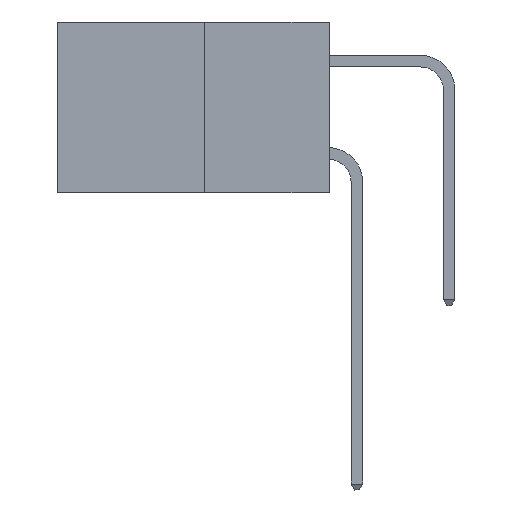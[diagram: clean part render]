
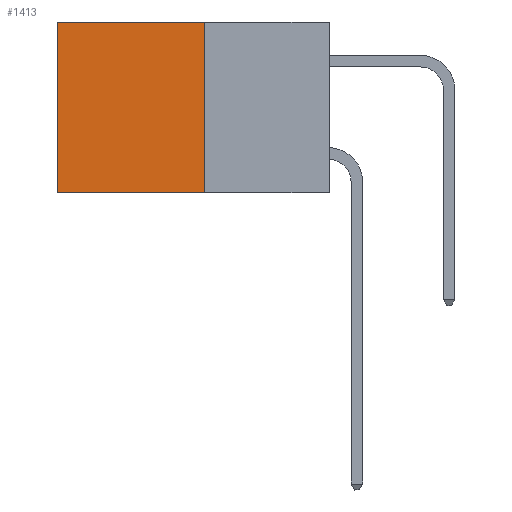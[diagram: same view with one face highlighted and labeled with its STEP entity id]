
A CAD part, left-side view. The second image highlights one B-rep face of the part: STEP entity #1413.
In plain terms, the highlighted planar face has unit normal (-1, 0, 0).
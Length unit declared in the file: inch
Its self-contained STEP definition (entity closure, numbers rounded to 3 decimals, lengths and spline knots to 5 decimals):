
#1413 = ADVANCED_FACE ( 'NONE', ( #7518 ), #26411, .F. ) ;
#2017 = EDGE_CURVE ( 'NONE', #8713, #20307, #16865, .T. ) ;
#4423 = ORIENTED_EDGE ( 'NONE', *, *, #18683, .T. ) ;
#5216 = VECTOR ( 'NONE', #16860, 39.37008 ) ;
#7518 = FACE_OUTER_BOUND ( 'NONE', #29210, .T. ) ;
#7617 = LINE ( 'NONE', #21825, #5216 ) ;
#8713 = VERTEX_POINT ( 'NONE', #15814 ) ;
#9788 = AXIS2_PLACEMENT_3D ( 'NONE', #26733, #26406, #26300 ) ;
#10083 = DIRECTION ( 'NONE',  ( 0., 1., 0. ) ) ;
#10238 = VECTOR ( 'NONE', #16153, 39.37008 ) ;
#10634 = EDGE_CURVE ( 'NONE', #20307, #26364, #30525, .T. ) ;
#14862 = CARTESIAN_POINT ( 'NONE',  ( 0.277, 0.59, -0.37 ) ) ;
#15399 = ORIENTED_EDGE ( 'NONE', *, *, #10634, .F. ) ;
#15814 = CARTESIAN_POINT ( 'NONE',  ( 0.277, 0.27, 0. ) ) ;
#16047 = CARTESIAN_POINT ( 'NONE',  ( 0.277, 0.27, -0.37 ) ) ;
#16144 = CARTESIAN_POINT ( 'NONE',  ( 0.277, 0.59, 0. ) ) ;
#16153 = DIRECTION ( 'NONE',  ( 0., 0., -1. ) ) ;
#16860 = DIRECTION ( 'NONE',  ( 0., 0., -1. ) ) ;
#16865 = LINE ( 'NONE', #16047, #10238 ) ;
#17134 = CARTESIAN_POINT ( 'NONE',  ( 0.277, 0.27, -0.37 ) ) ;
#17988 = VECTOR ( 'NONE', #10083, 39.37008 ) ;
#18683 = EDGE_CURVE ( 'NONE', #8713, #30378, #31106, .T. ) ;
#18717 = CARTESIAN_POINT ( 'NONE',  ( 0.277, 0.27, 0. ) ) ;
#19524 = EDGE_CURVE ( 'NONE', #30378, #26364, #7617, .T. ) ;
#20307 = VERTEX_POINT ( 'NONE', #17134 ) ;
#21789 = ORIENTED_EDGE ( 'NONE', *, *, #19524, .T. ) ;
#21825 = CARTESIAN_POINT ( 'NONE',  ( 0.277, 0.59, -0.37 ) ) ;
#23637 = VECTOR ( 'NONE', #28815, 39.37008 ) ;
#25001 = CARTESIAN_POINT ( 'NONE',  ( 0.277, 0.27, -0.37 ) ) ;
#26300 = DIRECTION ( 'NONE',  ( 0., 0., -1. ) ) ;
#26364 = VERTEX_POINT ( 'NONE', #14862 ) ;
#26406 = DIRECTION ( 'NONE',  ( 1., 0., 0. ) ) ;
#26411 = PLANE ( 'NONE',  #9788 ) ;
#26733 = CARTESIAN_POINT ( 'NONE',  ( 0.277, 0.27, -0.37 ) ) ;
#28815 = DIRECTION ( 'NONE',  ( 0., 1., 0. ) ) ;
#29210 = EDGE_LOOP ( 'NONE', ( #21789, #15399, #31426, #4423 ) ) ;
#30378 = VERTEX_POINT ( 'NONE', #16144 ) ;
#30525 = LINE ( 'NONE', #25001, #17988 ) ;
#31106 = LINE ( 'NONE', #18717, #23637 ) ;
#31426 = ORIENTED_EDGE ( 'NONE', *, *, #2017, .F. ) ;
